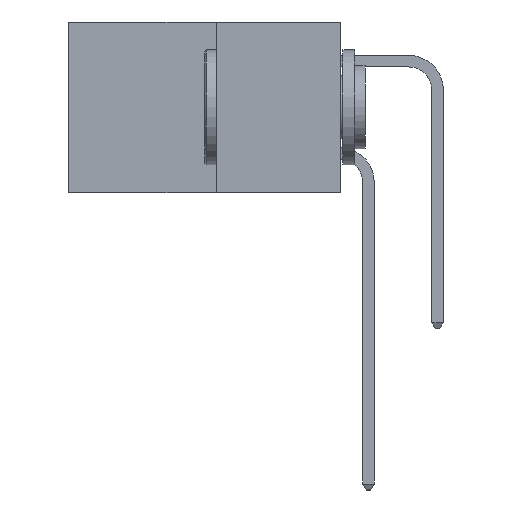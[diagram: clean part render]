
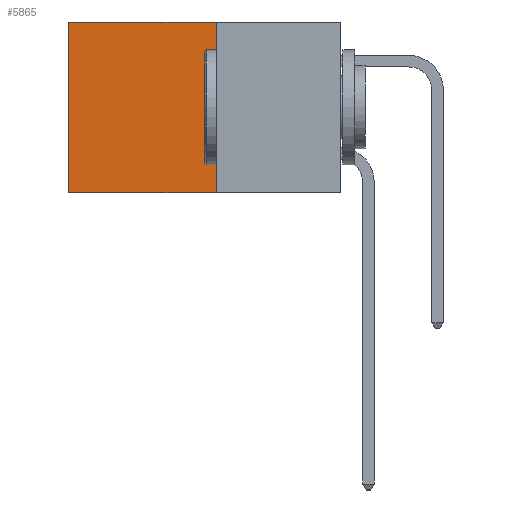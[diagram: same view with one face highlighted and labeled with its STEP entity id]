
A CAD part, left-side view. The second image highlights one B-rep face of the part: STEP entity #5865.
In plain terms, the highlighted planar face has unit normal (-1, 0, 0).
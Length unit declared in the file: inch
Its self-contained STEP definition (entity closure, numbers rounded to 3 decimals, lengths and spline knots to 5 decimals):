
#164 = VECTOR ( 'NONE', #6945, 39.37008 ) ;
#249 = VECTOR ( 'NONE', #11865, 39.37008 ) ;
#282 = VERTEX_POINT ( 'NONE', #4543 ) ;
#492 = CARTESIAN_POINT ( 'NONE',  ( 0.277, 0.27, -0.37 ) ) ;
#707 = ORIENTED_EDGE ( 'NONE', *, *, #1183, .F. ) ;
#711 = VECTOR ( 'NONE', #11688, 39.37008 ) ;
#1183 = EDGE_CURVE ( 'NONE', #5565, #1999, #8396, .T. ) ;
#1732 = VERTEX_POINT ( 'NONE', #4896 ) ;
#1999 = VERTEX_POINT ( 'NONE', #7669 ) ;
#2631 = EDGE_CURVE ( 'NONE', #282, #5565, #5959, .T. ) ;
#2651 = EDGE_CURVE ( 'NONE', #282, #1732, #5655, .T. ) ;
#3047 = CARTESIAN_POINT ( 'NONE',  ( 0.277, 0.27, -0.37 ) ) ;
#3183 = VECTOR ( 'NONE', #10253, 39.37008 ) ;
#4543 = CARTESIAN_POINT ( 'NONE',  ( 0.277, 0.27, 0. ) ) ;
#4896 = CARTESIAN_POINT ( 'NONE',  ( 0.277, 0.59, 0. ) ) ;
#5045 = AXIS2_PLACEMENT_3D ( 'NONE', #10424, #10120, #10070 ) ;
#5565 = VERTEX_POINT ( 'NONE', #492 ) ;
#5655 = LINE ( 'NONE', #11915, #3183 ) ;
#5689 = EDGE_LOOP ( 'NONE', ( #10670, #707, #5955, #8517 ) ) ;
#5865 = ADVANCED_FACE ( 'NONE', ( #6072 ), #10135, .F. ) ;
#5955 = ORIENTED_EDGE ( 'NONE', *, *, #2631, .F. ) ;
#5959 = LINE ( 'NONE', #11967, #711 ) ;
#6072 = FACE_OUTER_BOUND ( 'NONE', #5689, .T. ) ;
#6945 = DIRECTION ( 'NONE',  ( 0., 0., -1. ) ) ;
#7012 = CARTESIAN_POINT ( 'NONE',  ( 0.277, 0.59, -0.37 ) ) ;
#7669 = CARTESIAN_POINT ( 'NONE',  ( 0.277, 0.59, -0.37 ) ) ;
#7996 = EDGE_CURVE ( 'NONE', #1732, #1999, #8010, .T. ) ;
#8010 = LINE ( 'NONE', #7012, #164 ) ;
#8396 = LINE ( 'NONE', #3047, #249 ) ;
#8517 = ORIENTED_EDGE ( 'NONE', *, *, #2651, .T. ) ;
#10070 = DIRECTION ( 'NONE',  ( 0., 0., -1. ) ) ;
#10120 = DIRECTION ( 'NONE',  ( 1., 0., 0. ) ) ;
#10135 = PLANE ( 'NONE',  #5045 ) ;
#10253 = DIRECTION ( 'NONE',  ( 0., 1., 0. ) ) ;
#10424 = CARTESIAN_POINT ( 'NONE',  ( 0.277, 0.27, -0.37 ) ) ;
#10670 = ORIENTED_EDGE ( 'NONE', *, *, #7996, .T. ) ;
#11688 = DIRECTION ( 'NONE',  ( 0., 0., -1. ) ) ;
#11865 = DIRECTION ( 'NONE',  ( 0., 1., 0. ) ) ;
#11915 = CARTESIAN_POINT ( 'NONE',  ( 0.277, 0.27, 0. ) ) ;
#11967 = CARTESIAN_POINT ( 'NONE',  ( 0.277, 0.27, -0.37 ) ) ;
